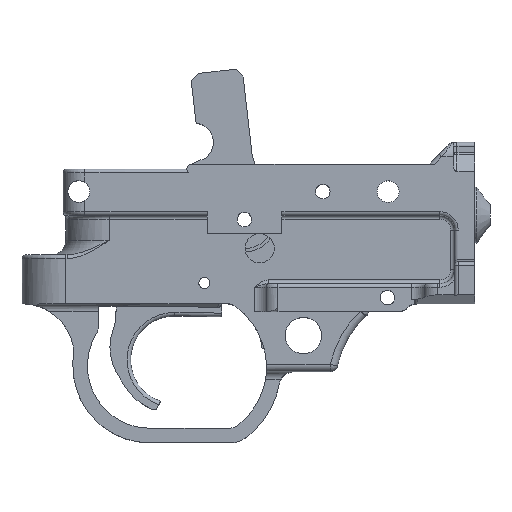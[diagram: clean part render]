
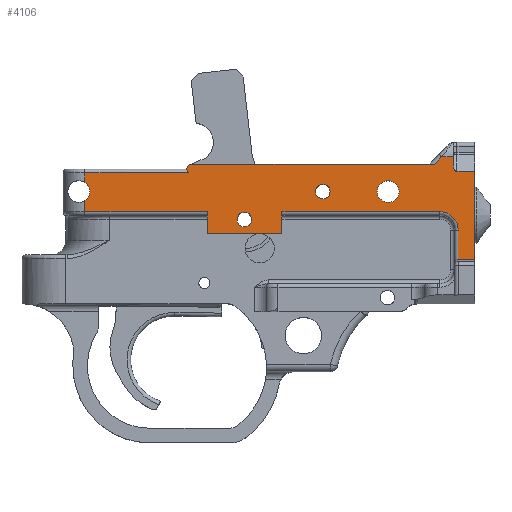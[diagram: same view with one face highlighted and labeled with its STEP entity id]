
A CAD part, top view. The second image highlights one B-rep face of the part: STEP entity #4106.
In plain terms, the highlighted planar face has unit normal (0, 0, 1).
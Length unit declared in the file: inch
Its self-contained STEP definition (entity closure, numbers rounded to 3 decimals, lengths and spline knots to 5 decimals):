
#3389=CARTESIAN_POINT('',(2.46491,0.70451,0.1325));
#3390=VERTEX_POINT('',#3389);
#3397=CARTESIAN_POINT('',(2.46491,-0.05399,0.1325));
#3398=VERTEX_POINT('',#3397);
#3399=CARTESIAN_POINT('',(2.46491,0.70451,0.1325));
#3400=DIRECTION('',(0.0,-1.0,0.0));
#3401=VECTOR('',#3400,0.7585);
#3402=LINE('',#3399,#3401);
#3403=EDGE_CURVE('',#3390,#3398,#3402,.T.);
#3703=CARTESIAN_POINT('',(0.03591,0.76701,0.1325));
#3704=VERTEX_POINT('',#3703);
#3711=CARTESIAN_POINT('',(2.1193,0.76701,0.1325));
#3712=VERTEX_POINT('',#3711);
#3713=CARTESIAN_POINT('',(0.03591,0.76701,0.1325));
#3714=DIRECTION('',(1.0,0.0,0.0));
#3715=VECTOR('',#3714,2.08339);
#3716=LINE('',#3713,#3715);
#3717=EDGE_CURVE('',#3704,#3712,#3716,.T.);
#3811=CARTESIAN_POINT('',(-0.88109,0.69376,0.1325));
#3812=VERTEX_POINT('',#3811);
#3885=CARTESIAN_POINT('',(0.00785,0.69376,0.1325));
#3886=VERTEX_POINT('',#3885);
#3911=CARTESIAN_POINT('',(-0.88109,0.69376,0.1325));
#3912=DIRECTION('',(1.0,0.0,0.0));
#3913=VECTOR('',#3912,0.88894);
#3914=LINE('',#3911,#3913);
#3915=EDGE_CURVE('',#3812,#3886,#3914,.T.);
#3920=CARTESIAN_POINT('',(2.46491,-0.05399,0.1325));
#3921=DIRECTION('',(0.0,0.0,-1.0));
#3922=DIRECTION('',(-1.0,0.0,0.0));
#3923=AXIS2_PLACEMENT_3D('',#3920,#3921,#3922);
#3924=PLANE('',#3923);
#3925=CARTESIAN_POINT('',(0.03591,0.72501,0.1325));
#3926=DIRECTION('',(0.0,0.0,-1.));
#3927=DIRECTION('',(-0.707,0.707,0.0));
#3928=AXIS2_PLACEMENT_3D('',#3925,#3926,#3927);
#3929=CIRCLE('',#3928,0.042);
#3930=EDGE_CURVE('',#3886,#3704,#3929,.T.);
#3931=ORIENTED_EDGE('',*,*,#3930,.F.);
#3932=ORIENTED_EDGE('',*,*,#3915,.F.);
#3933=CARTESIAN_POINT('',(-0.88109,0.60951,0.1325));
#3934=VERTEX_POINT('',#3933);
#3935=CARTESIAN_POINT('',(-0.88109,0.60951,0.1325));
#3936=DIRECTION('',(0.0,1.0,0.0));
#3937=VECTOR('',#3936,0.08425);
#3938=LINE('',#3935,#3937);
#3939=EDGE_CURVE('',#3934,#3812,#3938,.T.);
#3940=ORIENTED_EDGE('',*,*,#3939,.F.);
#3941=CARTESIAN_POINT('',(-0.88109,0.45451,0.1325));
#3942=VERTEX_POINT('',#3941);
#3943=CARTESIAN_POINT('',(-0.93384,0.53201,0.1325));
#3944=DIRECTION('',(0.0,0.0,1.0));
#3945=DIRECTION('',(1.0,0.0,0.0));
#3946=AXIS2_PLACEMENT_3D('',#3943,#3944,#3945);
#3947=CIRCLE('',#3946,0.09375);
#3948=EDGE_CURVE('',#3942,#3934,#3947,.T.);
#3949=ORIENTED_EDGE('',*,*,#3948,.F.);
#3950=CARTESIAN_POINT('',(-0.88109,0.35826,0.1325));
#3951=VERTEX_POINT('',#3950);
#3952=CARTESIAN_POINT('',(-0.88109,0.35826,0.1325));
#3953=DIRECTION('',(0.0,1.0,0.0));
#3954=VECTOR('',#3953,0.09625);
#3955=LINE('',#3952,#3954);
#3956=EDGE_CURVE('',#3951,#3942,#3955,.T.);
#3957=ORIENTED_EDGE('',*,*,#3956,.F.);
#3958=CARTESIAN_POINT('',(0.16941,0.35826,0.1325));
#3959=VERTEX_POINT('',#3958);
#3960=CARTESIAN_POINT('',(0.16941,0.35826,0.1325));
#3961=DIRECTION('',(-1.0,0.0,0.0));
#3962=VECTOR('',#3961,1.0505);
#3963=LINE('',#3960,#3962);
#3964=EDGE_CURVE('',#3959,#3951,#3963,.T.);
#3965=ORIENTED_EDGE('',*,*,#3964,.F.);
#3966=CARTESIAN_POINT('',(0.16941,0.17001,0.1325));
#3967=VERTEX_POINT('',#3966);
#3968=CARTESIAN_POINT('',(0.16941,0.35826,0.1325));
#3969=DIRECTION('',(0.0,-1.0,0.0));
#3970=VECTOR('',#3969,0.18825);
#3971=LINE('',#3968,#3970);
#3972=EDGE_CURVE('',#3959,#3967,#3971,.T.);
#3973=ORIENTED_EDGE('',*,*,#3972,.T.);
#3974=CARTESIAN_POINT('',(0.81041,0.17001,0.1325));
#3975=VERTEX_POINT('',#3974);
#3976=CARTESIAN_POINT('',(0.16941,0.17001,0.1325));
#3977=DIRECTION('',(1.0,0.0,0.0));
#3978=VECTOR('',#3977,0.641);
#3979=LINE('',#3976,#3978);
#3980=EDGE_CURVE('',#3967,#3975,#3979,.T.);
#3981=ORIENTED_EDGE('',*,*,#3980,.T.);
#3982=CARTESIAN_POINT('',(0.81041,0.35826,0.1325));
#3983=VERTEX_POINT('',#3982);
#3984=CARTESIAN_POINT('',(0.81041,0.17001,0.1325));
#3985=DIRECTION('',(0.0,1.0,0.0));
#3986=VECTOR('',#3985,0.18825);
#3987=LINE('',#3984,#3986);
#3988=EDGE_CURVE('',#3975,#3983,#3987,.T.);
#3989=ORIENTED_EDGE('',*,*,#3988,.T.);
#3990=CARTESIAN_POINT('',(2.16591,0.35826,0.1325));
#3991=VERTEX_POINT('',#3990);
#3992=CARTESIAN_POINT('',(2.16591,0.35826,0.1325));
#3993=DIRECTION('',(-1.0,0.0,0.0));
#3994=VECTOR('',#3993,1.3555);
#3995=LINE('',#3992,#3994);
#3996=EDGE_CURVE('',#3991,#3983,#3995,.T.);
#3997=ORIENTED_EDGE('',*,*,#3996,.F.);
#3998=CARTESIAN_POINT('',(2.32216,0.20201,0.1325));
#3999=VERTEX_POINT('',#3998);
#4000=CARTESIAN_POINT('',(2.16591,0.20201,0.1325));
#4001=DIRECTION('',(0.0,0.0,1.0));
#4002=DIRECTION('',(0.707,0.707,0.0));
#4003=AXIS2_PLACEMENT_3D('',#4000,#4001,#4002);
#4004=CIRCLE('',#4003,0.15625);
#4005=EDGE_CURVE('',#3999,#3991,#4004,.T.);
#4006=ORIENTED_EDGE('',*,*,#4005,.F.);
#4007=CARTESIAN_POINT('',(2.32216,-0.05399,0.1325));
#4008=VERTEX_POINT('',#4007);
#4009=CARTESIAN_POINT('',(2.32216,-0.05399,0.1325));
#4010=DIRECTION('',(0.0,1.0,0.0));
#4011=VECTOR('',#4010,0.256);
#4012=LINE('',#4009,#4011);
#4013=EDGE_CURVE('',#4008,#3999,#4012,.T.);
#4014=ORIENTED_EDGE('',*,*,#4013,.F.);
#4015=CARTESIAN_POINT('',(2.32216,-0.05399,0.1325));
#4016=VERTEX_POINT('',#4015);
#4017=CARTESIAN_POINT('',(2.32216,-0.08561,0.1325));
#4018=DIRECTION('',(0.0,0.0,-1.0));
#4019=DIRECTION('',(0.0,1.0,0.0));
#4020=AXIS2_PLACEMENT_3D('',#4017,#4018,#4019);
#4021=ELLIPSE('',#4020,0.03163,0.03125);
#4022=EDGE_CURVE('',#4016,#4008,#4021,.F.);
#4023=ORIENTED_EDGE('',*,*,#4022,.F.);
#4024=CARTESIAN_POINT('',(2.46491,-0.05399,0.1325));
#4025=DIRECTION('',(-1.0,0.0,0.0));
#4026=VECTOR('',#4025,0.14275);
#4027=LINE('',#4024,#4026);
#4028=EDGE_CURVE('',#3398,#4016,#4027,.T.);
#4029=ORIENTED_EDGE('',*,*,#4028,.F.);
#4030=ORIENTED_EDGE('',*,*,#3403,.F.);
#4031=CARTESIAN_POINT('',(2.31216,0.70451,0.1325));
#4032=VERTEX_POINT('',#4031);
#4033=CARTESIAN_POINT('',(2.46491,0.70451,0.1325));
#4034=DIRECTION('',(-1.0,0.0,0.0));
#4035=VECTOR('',#4034,0.15275);
#4036=LINE('',#4033,#4035);
#4037=EDGE_CURVE('',#3390,#4032,#4036,.T.);
#4038=ORIENTED_EDGE('',*,*,#4037,.T.);
#4039=CARTESIAN_POINT('',(2.28091,0.75172,0.1325));
#4040=VERTEX_POINT('',#4039);
#4041=CARTESIAN_POINT('',(2.31216,0.75172,0.1325));
#4042=DIRECTION('',(0.0,0.0,1.0));
#4043=DIRECTION('',(0.0,-1.0,0.0));
#4044=AXIS2_PLACEMENT_3D('',#4041,#4042,#4043);
#4045=ELLIPSE('',#4044,0.04721,0.03125);
#4046=EDGE_CURVE('',#4040,#4032,#4045,.T.);
#4047=ORIENTED_EDGE('',*,*,#4046,.F.);
#4048=CARTESIAN_POINT('',(2.28091,0.82951,0.1325));
#4049=VERTEX_POINT('',#4048);
#4050=CARTESIAN_POINT('',(2.28091,0.75172,0.1325));
#4051=DIRECTION('',(0.0,1.0,0.0));
#4052=VECTOR('',#4051,0.07779);
#4053=LINE('',#4050,#4052);
#4054=EDGE_CURVE('',#4040,#4049,#4053,.T.);
#4055=ORIENTED_EDGE('',*,*,#4054,.T.);
#4056=CARTESIAN_POINT('',(2.1818,0.82951,0.1325));
#4057=VERTEX_POINT('',#4056);
#4058=CARTESIAN_POINT('',(2.1818,0.82951,0.1325));
#4059=DIRECTION('',(1.0,0.0,0.0));
#4060=VECTOR('',#4059,0.09911);
#4061=LINE('',#4058,#4060);
#4062=EDGE_CURVE('',#4057,#4049,#4061,.T.);
#4063=ORIENTED_EDGE('',*,*,#4062,.F.);
#4064=CARTESIAN_POINT('',(2.1193,0.76701,0.1325));
#4065=DIRECTION('',(0.707,0.707,0.0));
#4066=VECTOR('',#4065,0.08839);
#4067=LINE('',#4064,#4066);
#4068=EDGE_CURVE('',#3712,#4057,#4067,.T.);
#4069=ORIENTED_EDGE('',*,*,#4068,.F.);
#4070=ORIENTED_EDGE('',*,*,#3717,.F.);
#4071=EDGE_LOOP('',(#3931,#3932,#3940,#3949,#3957,#3965,#3973,#3981,#3989,#3997,#4006,#4014,#4023,#4029,#4030,#4038,#4047,#4055,#4063,#4069,#4070));
#4072=FACE_OUTER_BOUND('',#4071,.T.);
#4073=CARTESIAN_POINT('',(0.55041,0.29201,0.1325));
#4074=VERTEX_POINT('',#4073);
#4075=CARTESIAN_POINT('',(0.48791,0.29201,0.1325));
#4076=DIRECTION('',(0.0,0.0,-1.0));
#4077=DIRECTION('',(1.0,0.0,0.0));
#4078=AXIS2_PLACEMENT_3D('',#4075,#4076,#4077);
#4079=CIRCLE('',#4078,0.0625);
#4080=EDGE_CURVE('',#4074,#4074,#4079,.T.);
#4081=ORIENTED_EDGE('',*,*,#4080,.T.);
#4082=EDGE_LOOP('',(#4081));
#4083=FACE_BOUND('',#4082,.T.);
#4084=CARTESIAN_POINT('',(1.22341,0.53201,0.1325));
#4085=VERTEX_POINT('',#4084);
#4086=CARTESIAN_POINT('',(1.16091,0.53201,0.1325));
#4087=DIRECTION('',(0.0,0.0,-1.0));
#4088=DIRECTION('',(1.0,0.0,0.0));
#4089=AXIS2_PLACEMENT_3D('',#4086,#4087,#4088);
#4090=CIRCLE('',#4089,0.0625);
#4091=EDGE_CURVE('',#4085,#4085,#4090,.T.);
#4092=ORIENTED_EDGE('',*,*,#4091,.T.);
#4093=EDGE_LOOP('',(#4092));
#4094=FACE_BOUND('',#4093,.T.);
#4095=CARTESIAN_POINT('',(1.62741,0.53201,0.1325));
#4096=VERTEX_POINT('',#4095);
#4097=CARTESIAN_POINT('',(1.72116,0.53201,0.1325));
#4098=DIRECTION('',(0.0,0.0,1.0));
#4099=DIRECTION('',(1.0,0.0,0.0));
#4100=AXIS2_PLACEMENT_3D('',#4097,#4098,#4099);
#4101=CIRCLE('',#4100,0.09375);
#4102=EDGE_CURVE('',#4096,#4096,#4101,.T.);
#4103=ORIENTED_EDGE('',*,*,#4102,.F.);
#4104=EDGE_LOOP('',(#4103));
#4105=FACE_BOUND('',#4104,.T.);
#4106=ADVANCED_FACE('',(#4072,#4083,#4094,#4105),#3924,.F.);
